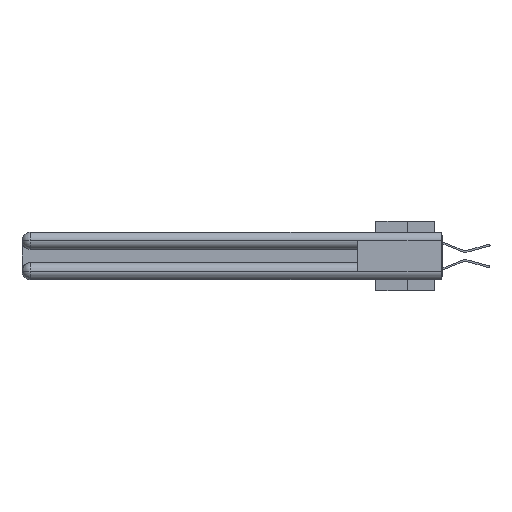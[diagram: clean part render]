
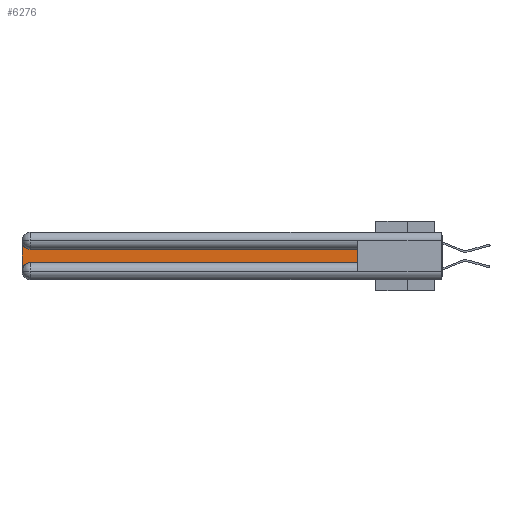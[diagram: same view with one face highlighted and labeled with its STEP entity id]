
A CAD part, left-side view. The second image highlights one B-rep face of the part: STEP entity #6276.
In plain terms, the highlighted planar face has unit normal (-1, 0, 0).
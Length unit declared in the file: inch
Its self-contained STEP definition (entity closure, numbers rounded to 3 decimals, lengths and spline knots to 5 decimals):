
#1365 = AXIS2_PLACEMENT_3D ( 'NONE', #20626, #34938, #20809 ) ;
#1401 = VERTEX_POINT ( 'NONE', #13317 ) ;
#1403 = CIRCLE ( 'NONE', #13117, 0.06 ) ;
#3485 = DIRECTION ( 'NONE',  ( 0., 0., -1. ) ) ;
#3579 = DIRECTION ( 'NONE',  ( 0., -1., 0. ) ) ;
#4235 = CARTESIAN_POINT ( 'NONE',  ( 0.075, 3., -0.2175 ) ) ;
#4457 = EDGE_CURVE ( 'NONE', #36180, #9442, #28207, .T. ) ;
#5193 = VECTOR ( 'NONE', #3579, 39.37008 ) ;
#5848 = EDGE_CURVE ( 'NONE', #1401, #35296, #1403, .T. ) ;
#5861 = VECTOR ( 'NONE', #16590, 39.37008 ) ;
#6007 = CARTESIAN_POINT ( 'NONE',  ( 0.075, 0.6, -0.2175 ) ) ;
#6276 = ADVANCED_FACE ( 'NONE', ( #9438 ), #34759, .F. ) ;
#6771 = CARTESIAN_POINT ( 'NONE',  ( 0.075, 0.6, -0.2175 ) ) ;
#6864 = CARTESIAN_POINT ( 'NONE',  ( 0.075, 2.94, -0.1225 ) ) ;
#7112 = DIRECTION ( 'NONE',  ( 1., 0., 0. ) ) ;
#8566 = DIRECTION ( 'NONE',  ( 0., 0., 1. ) ) ;
#8884 = EDGE_LOOP ( 'NONE', ( #29149, #29767, #35870, #26590, #17381, #34269 ) ) ;
#9354 = CARTESIAN_POINT ( 'NONE',  ( 0.075, 2.94, -0.2775 ) ) ;
#9438 = FACE_OUTER_BOUND ( 'NONE', #8884, .T. ) ;
#9442 = VERTEX_POINT ( 'NONE', #18705 ) ;
#10235 = CARTESIAN_POINT ( 'NONE',  ( 0.075, 2.94, -0.0625 ) ) ;
#11736 = CIRCLE ( 'NONE', #21700, 0.06 ) ;
#13117 = AXIS2_PLACEMENT_3D ( 'NONE', #9354, #31201, #3485 ) ;
#13317 = CARTESIAN_POINT ( 'NONE',  ( 0.075, 3., -0.2775 ) ) ;
#14871 = LINE ( 'NONE', #4235, #23919 ) ;
#14953 = EDGE_CURVE ( 'NONE', #24723, #1401, #14871, .T. ) ;
#16590 = DIRECTION ( 'NONE',  ( 0., 1., 0. ) ) ;
#17001 = CARTESIAN_POINT ( 'NONE',  ( 0.075, 2.94, -0.2175 ) ) ;
#17381 = ORIENTED_EDGE ( 'NONE', *, *, #32619, .T. ) ;
#17701 = CARTESIAN_POINT ( 'NONE',  ( 0.075, 0.6, -0.2175 ) ) ;
#18478 = DIRECTION ( 'NONE',  ( 0., 0., -1. ) ) ;
#18705 = CARTESIAN_POINT ( 'NONE',  ( 0.075, 0.6, -0.1225 ) ) ;
#19519 = CARTESIAN_POINT ( 'NONE',  ( 0.075, 0.6, -0.1225 ) ) ;
#19994 = VERTEX_POINT ( 'NONE', #6864 ) ;
#20626 = CARTESIAN_POINT ( 'NONE',  ( 0.075, 3., -0.1225 ) ) ;
#20634 = LINE ( 'NONE', #17701, #5193 ) ;
#20809 = DIRECTION ( 'NONE',  ( 0., 0., -1. ) ) ;
#21700 = AXIS2_PLACEMENT_3D ( 'NONE', #10235, #7112, #18478 ) ;
#22630 = LINE ( 'NONE', #19519, #5861 ) ;
#22910 = EDGE_CURVE ( 'NONE', #19994, #24723, #11736, .T. ) ;
#23261 = VECTOR ( 'NONE', #8566, 39.37008 ) ;
#23490 = DIRECTION ( 'NONE',  ( 0., 0., -1. ) ) ;
#23919 = VECTOR ( 'NONE', #23490, 39.37008 ) ;
#24723 = VERTEX_POINT ( 'NONE', #35225 ) ;
#26590 = ORIENTED_EDGE ( 'NONE', *, *, #5848, .T. ) ;
#28207 = LINE ( 'NONE', #6007, #23261 ) ;
#29149 = ORIENTED_EDGE ( 'NONE', *, *, #33866, .T. ) ;
#29767 = ORIENTED_EDGE ( 'NONE', *, *, #22910, .T. ) ;
#31201 = DIRECTION ( 'NONE',  ( 1., 0., 0. ) ) ;
#32619 = EDGE_CURVE ( 'NONE', #35296, #36180, #20634, .T. ) ;
#33866 = EDGE_CURVE ( 'NONE', #9442, #19994, #22630, .T. ) ;
#34269 = ORIENTED_EDGE ( 'NONE', *, *, #4457, .T. ) ;
#34759 = PLANE ( 'NONE',  #1365 ) ;
#34938 = DIRECTION ( 'NONE',  ( 1., 0., 0. ) ) ;
#35225 = CARTESIAN_POINT ( 'NONE',  ( 0.075, 3., -0.0625 ) ) ;
#35296 = VERTEX_POINT ( 'NONE', #17001 ) ;
#35870 = ORIENTED_EDGE ( 'NONE', *, *, #14953, .T. ) ;
#36180 = VERTEX_POINT ( 'NONE', #6771 ) ;
